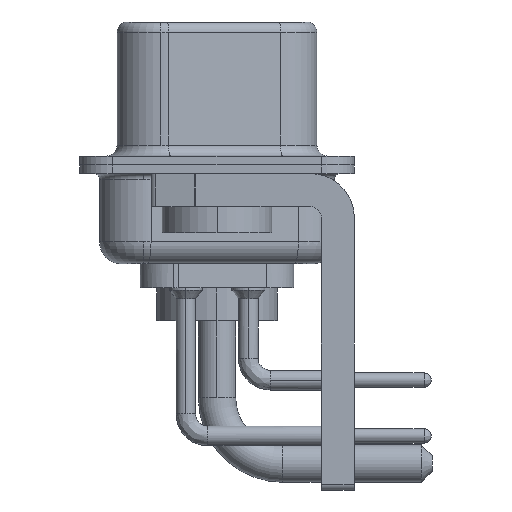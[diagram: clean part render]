
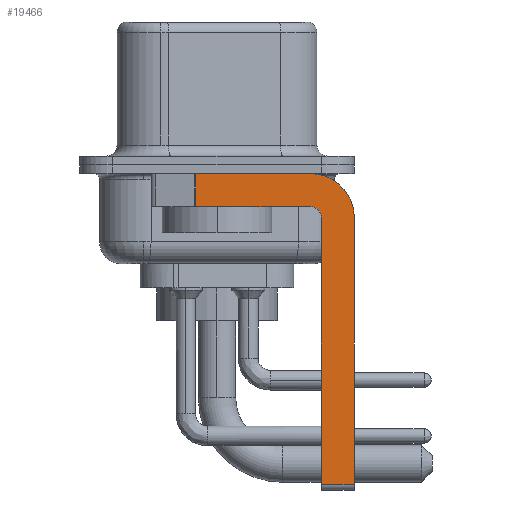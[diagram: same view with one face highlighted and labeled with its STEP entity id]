
A CAD part, left-side view. The second image highlights one B-rep face of the part: STEP entity #19466.
In plain terms, the highlighted planar face has unit normal (-1, 0, 0).
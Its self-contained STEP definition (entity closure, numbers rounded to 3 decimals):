
#228 = VECTOR ( 'NONE', #19815, 1000. ) ;
#317 = CARTESIAN_POINT ( 'NONE',  ( -2.9, 3., -0.4 ) ) ;
#423 = VERTEX_POINT ( 'NONE', #6134 ) ;
#1261 = VERTEX_POINT ( 'NONE', #2468 ) ;
#1578 = EDGE_CURVE ( 'NONE', #4533, #2920, #12346, .T. ) ;
#1702 = ORIENTED_EDGE ( 'NONE', *, *, #6031, .F. ) ;
#1703 = DIRECTION ( 'NONE',  ( 1., 0., 0. ) ) ;
#2169 = DIRECTION ( 'NONE',  ( 0., 1., 0. ) ) ;
#2296 = CARTESIAN_POINT ( 'NONE',  ( -2.9, -4.25, -0.4 ) ) ;
#2468 = CARTESIAN_POINT ( 'NONE',  ( -2.9, -4.75, -14.55 ) ) ;
#2920 = VERTEX_POINT ( 'NONE', #18143 ) ;
#3136 = ORIENTED_EDGE ( 'NONE', *, *, #10582, .T. ) ;
#3227 = CARTESIAN_POINT ( 'NONE',  ( -2.9, -4.25, -14.55 ) ) ;
#3310 = FACE_OUTER_BOUND ( 'NONE', #3607, .T. ) ;
#3601 = CARTESIAN_POINT ( 'NONE',  ( -2.9, -4.25, -1.9 ) ) ;
#3604 = DIRECTION ( 'NONE',  ( 0., 0., 1. ) ) ;
#3607 = EDGE_LOOP ( 'NONE', ( #9689, #3136, #16914, #15252, #1702, #12425, #17859, #3745 ) ) ;
#3643 = VERTEX_POINT ( 'NONE', #2296 ) ;
#3745 = ORIENTED_EDGE ( 'NONE', *, *, #17765, .F. ) ;
#3924 = VERTEX_POINT ( 'NONE', #10165 ) ;
#4294 = AXIS2_PLACEMENT_3D ( 'NONE', #14535, #1703, #8363 ) ;
#4533 = VERTEX_POINT ( 'NONE', #14181 ) ;
#5088 = LINE ( 'NONE', #3227, #13148 ) ;
#5336 = CARTESIAN_POINT ( 'NONE',  ( -2.9, 0.978, -0.4 ) ) ;
#5588 = CARTESIAN_POINT ( 'NONE',  ( -2.9, -6.25, -2.4 ) ) ;
#6031 = EDGE_CURVE ( 'NONE', #1261, #4533, #17674, .T. ) ;
#6134 = CARTESIAN_POINT ( 'NONE',  ( -2.9, -6.25, -14.55 ) ) ;
#6190 = CARTESIAN_POINT ( 'NONE',  ( -2.9, -4.25, -2.4 ) ) ;
#6567 = CARTESIAN_POINT ( 'NONE',  ( -2.9, -4.25, -2.4 ) ) ;
#7171 = VECTOR ( 'NONE', #11738, 1000. ) ;
#7534 = VECTOR ( 'NONE', #2169, 1000. ) ;
#8158 = EDGE_CURVE ( 'NONE', #2920, #3924, #14804, .T. ) ;
#8363 = DIRECTION ( 'NONE',  ( 0., 0., -1. ) ) ;
#9689 = ORIENTED_EDGE ( 'NONE', *, *, #15035, .F. ) ;
#9783 = DIRECTION ( 'NONE',  ( 0., -1., 0. ) ) ;
#10165 = CARTESIAN_POINT ( 'NONE',  ( -2.9, 0.978, -1.9 ) ) ;
#10582 = EDGE_CURVE ( 'NONE', #15554, #3924, #13578, .T. ) ;
#10797 = VERTEX_POINT ( 'NONE', #17648 ) ;
#10824 = CIRCLE ( 'NONE', #4294, 2. ) ;
#11310 = DIRECTION ( 'NONE',  ( 1., 0., 0. ) ) ;
#11511 = DIRECTION ( 'NONE',  ( 0., -1., 0. ) ) ;
#11738 = DIRECTION ( 'NONE',  ( 0., 0., -1. ) ) ;
#12346 = CIRCLE ( 'NONE', #16616, 0.5 ) ;
#12425 = ORIENTED_EDGE ( 'NONE', *, *, #16512, .T. ) ;
#13148 = VECTOR ( 'NONE', #9783, 1000. ) ;
#13193 = AXIS2_PLACEMENT_3D ( 'NONE', #6190, #11310, #18799 ) ;
#13578 = LINE ( 'NONE', #18280, #228 ) ;
#14181 = CARTESIAN_POINT ( 'NONE',  ( -2.9, -4.75, -2.4 ) ) ;
#14192 = CARTESIAN_POINT ( 'NONE',  ( -2.9, -4.75, -14.8 ) ) ;
#14393 = LINE ( 'NONE', #317, #18345 ) ;
#14467 = DIRECTION ( 'NONE',  ( -1., 0., 0. ) ) ;
#14535 = CARTESIAN_POINT ( 'NONE',  ( -2.9, -4.25, -2.4 ) ) ;
#14659 = EDGE_CURVE ( 'NONE', #10797, #423, #16871, .T. ) ;
#14804 = LINE ( 'NONE', #3601, #7534 ) ;
#15035 = EDGE_CURVE ( 'NONE', #15554, #3643, #14393, .T. ) ;
#15252 = ORIENTED_EDGE ( 'NONE', *, *, #1578, .F. ) ;
#15554 = VERTEX_POINT ( 'NONE', #5336 ) ;
#15935 = PLANE ( 'NONE',  #13193 ) ;
#16512 = EDGE_CURVE ( 'NONE', #1261, #423, #5088, .T. ) ;
#16616 = AXIS2_PLACEMENT_3D ( 'NONE', #6567, #14467, #18760 ) ;
#16871 = LINE ( 'NONE', #5588, #7171 ) ;
#16914 = ORIENTED_EDGE ( 'NONE', *, *, #8158, .F. ) ;
#17648 = CARTESIAN_POINT ( 'NONE',  ( -2.9, -6.25, -2.4 ) ) ;
#17674 = LINE ( 'NONE', #14192, #19782 ) ;
#17765 = EDGE_CURVE ( 'NONE', #3643, #10797, #10824, .T. ) ;
#17859 = ORIENTED_EDGE ( 'NONE', *, *, #14659, .F. ) ;
#18143 = CARTESIAN_POINT ( 'NONE',  ( -2.9, -4.25, -1.9 ) ) ;
#18280 = CARTESIAN_POINT ( 'NONE',  ( -2.9, 0.978, -1.9 ) ) ;
#18345 = VECTOR ( 'NONE', #11511, 1000. ) ;
#18760 = DIRECTION ( 'NONE',  ( 0., 0., 1. ) ) ;
#18799 = DIRECTION ( 'NONE',  ( 0., 0., -1. ) ) ;
#19466 = ADVANCED_FACE ( 'NONE', ( #3310 ), #15935, .F. ) ;
#19782 = VECTOR ( 'NONE', #3604, 1000. ) ;
#19815 = DIRECTION ( 'NONE',  ( 0., 0., -1. ) ) ;
